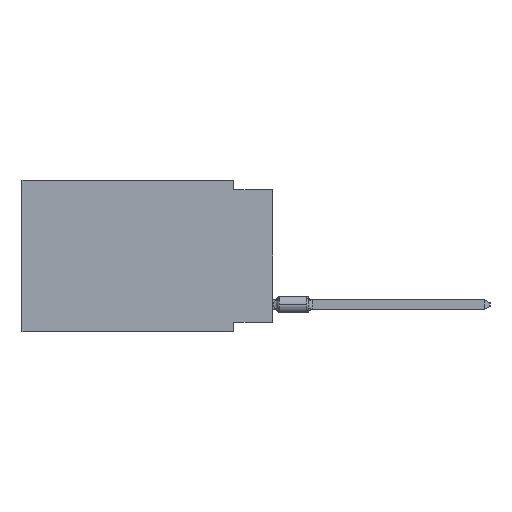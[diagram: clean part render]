
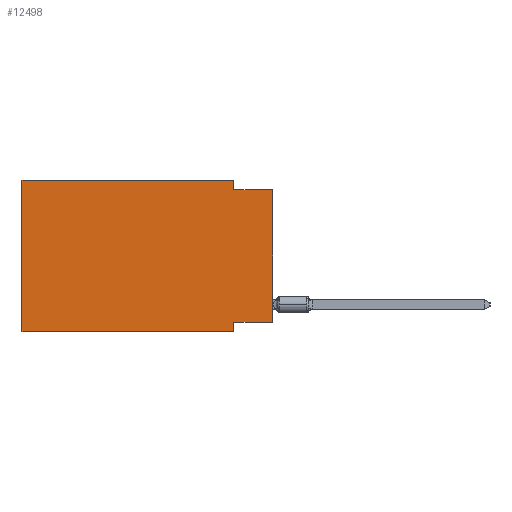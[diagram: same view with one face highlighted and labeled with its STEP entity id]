
A CAD part, left-side view. The second image highlights one B-rep face of the part: STEP entity #12498.
In plain terms, the highlighted planar face has unit normal (-1, 0, 0).
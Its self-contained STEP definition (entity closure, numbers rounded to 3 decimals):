
#252 = LINE ( 'NONE', #31422, #14810 ) ;
#639 = CARTESIAN_POINT ( 'NONE',  ( 0., 16.383, 0. ) ) ;
#1643 = LINE ( 'NONE', #35032, #6355 ) ;
#2842 = AXIS2_PLACEMENT_3D ( 'NONE', #639, #9046, #6292 ) ;
#3818 = DIRECTION ( 'NONE',  ( 0., 0., -1. ) ) ;
#5182 = VERTEX_POINT ( 'NONE', #30270 ) ;
#6174 = VERTEX_POINT ( 'NONE', #26324 ) ;
#6292 = DIRECTION ( 'NONE',  ( 0., 0., -1. ) ) ;
#6355 = VECTOR ( 'NONE', #26293, 1000. ) ;
#6793 = ORIENTED_EDGE ( 'NONE', *, *, #24753, .T. ) ;
#7084 = CARTESIAN_POINT ( 'NONE',  ( 0., 16.383, 0. ) ) ;
#7094 = VECTOR ( 'NONE', #14282, 1000. ) ;
#7994 = EDGE_CURVE ( 'NONE', #6174, #13652, #1643, .T. ) ;
#8576 = CARTESIAN_POINT ( 'NONE',  ( 0., 16.383, -9.906 ) ) ;
#9046 = DIRECTION ( 'NONE',  ( 1., 0., 0. ) ) ;
#9536 = VECTOR ( 'NONE', #25467, 1000. ) ;
#9659 = CARTESIAN_POINT ( 'NONE',  ( 0., 2.54, 0. ) ) ;
#10938 = DIRECTION ( 'NONE',  ( 0., -1., 0. ) ) ;
#11480 = ORIENTED_EDGE ( 'NONE', *, *, #14265, .F. ) ;
#12498 = ADVANCED_FACE ( 'NONE', ( #25291 ), #28547, .F. ) ;
#12613 = EDGE_CURVE ( 'NONE', #27181, #19630, #31659, .T. ) ;
#13433 = CARTESIAN_POINT ( 'NONE',  ( 0., 0., -9.271 ) ) ;
#13652 = VERTEX_POINT ( 'NONE', #7084 ) ;
#13937 = VECTOR ( 'NONE', #14886, 1000. ) ;
#14265 = EDGE_CURVE ( 'NONE', #13652, #34003, #33503, .T. ) ;
#14282 = DIRECTION ( 'NONE',  ( 0., -1., 0. ) ) ;
#14708 = EDGE_CURVE ( 'NONE', #27181, #14976, #252, .T. ) ;
#14810 = VECTOR ( 'NONE', #22501, 1000. ) ;
#14886 = DIRECTION ( 'NONE',  ( 0., 0., 1. ) ) ;
#14976 = VERTEX_POINT ( 'NONE', #30122 ) ;
#15390 = EDGE_LOOP ( 'NONE', ( #20135, #17851, #17297, #11480, #23582, #6793, #24641, #29841 ) ) ;
#15888 = CARTESIAN_POINT ( 'NONE',  ( 0., 0., -0.635 ) ) ;
#17000 = LINE ( 'NONE', #17716, #7094 ) ;
#17072 = CARTESIAN_POINT ( 'NONE',  ( 0., 16.383, 0. ) ) ;
#17297 = ORIENTED_EDGE ( 'NONE', *, *, #26036, .F. ) ;
#17716 = CARTESIAN_POINT ( 'NONE',  ( 0., 0., -0.635 ) ) ;
#17785 = CARTESIAN_POINT ( 'NONE',  ( 0., 0., 0. ) ) ;
#17851 = ORIENTED_EDGE ( 'NONE', *, *, #18271, .F. ) ;
#18271 = EDGE_CURVE ( 'NONE', #5182, #19630, #17000, .T. ) ;
#19630 = VERTEX_POINT ( 'NONE', #15888 ) ;
#19725 = EDGE_CURVE ( 'NONE', #14976, #21931, #28274, .T. ) ;
#20135 = ORIENTED_EDGE ( 'NONE', *, *, #12613, .T. ) ;
#20398 = LINE ( 'NONE', #23322, #35727 ) ;
#21931 = VERTEX_POINT ( 'NONE', #30150 ) ;
#22501 = DIRECTION ( 'NONE',  ( 0., 1., 0. ) ) ;
#23322 = CARTESIAN_POINT ( 'NONE',  ( 0., 2.54, 0. ) ) ;
#23582 = ORIENTED_EDGE ( 'NONE', *, *, #7994, .F. ) ;
#24641 = ORIENTED_EDGE ( 'NONE', *, *, #19725, .F. ) ;
#24753 = EDGE_CURVE ( 'NONE', #6174, #21931, #33570, .T. ) ;
#25183 = CARTESIAN_POINT ( 'NONE',  ( 0., 2.54, -9.906 ) ) ;
#25223 = VECTOR ( 'NONE', #10938, 1000. ) ;
#25291 = FACE_OUTER_BOUND ( 'NONE', #15390, .T. ) ;
#25467 = DIRECTION ( 'NONE',  ( 0., -1., 0. ) ) ;
#26036 = EDGE_CURVE ( 'NONE', #34003, #5182, #20398, .T. ) ;
#26293 = DIRECTION ( 'NONE',  ( 0., 0., 1. ) ) ;
#26324 = CARTESIAN_POINT ( 'NONE',  ( 0., 16.383, -9.906 ) ) ;
#27181 = VERTEX_POINT ( 'NONE', #13433 ) ;
#28274 = LINE ( 'NONE', #25183, #32068 ) ;
#28445 = DIRECTION ( 'NONE',  ( 0., 0., -1. ) ) ;
#28547 = PLANE ( 'NONE',  #2842 ) ;
#29841 = ORIENTED_EDGE ( 'NONE', *, *, #14708, .F. ) ;
#30122 = CARTESIAN_POINT ( 'NONE',  ( 0., 2.54, -9.271 ) ) ;
#30150 = CARTESIAN_POINT ( 'NONE',  ( 0., 2.54, -9.906 ) ) ;
#30270 = CARTESIAN_POINT ( 'NONE',  ( 0., 2.54, -0.635 ) ) ;
#31422 = CARTESIAN_POINT ( 'NONE',  ( 0., 0., -9.271 ) ) ;
#31659 = LINE ( 'NONE', #17785, #13937 ) ;
#32068 = VECTOR ( 'NONE', #28445, 1000. ) ;
#33503 = LINE ( 'NONE', #17072, #9536 ) ;
#33570 = LINE ( 'NONE', #8576, #25223 ) ;
#34003 = VERTEX_POINT ( 'NONE', #9659 ) ;
#35032 = CARTESIAN_POINT ( 'NONE',  ( 0., 16.383, 0. ) ) ;
#35727 = VECTOR ( 'NONE', #3818, 1000. ) ;
